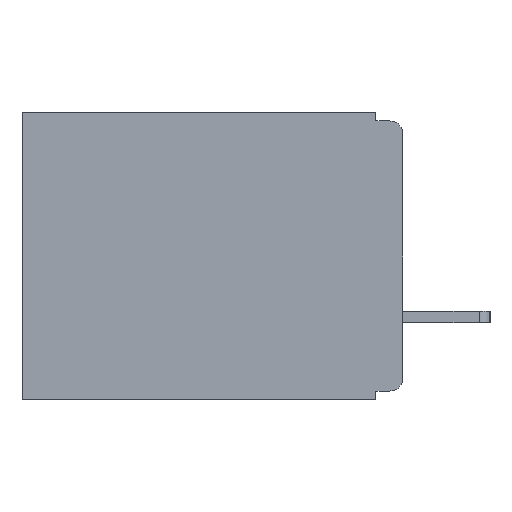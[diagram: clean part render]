
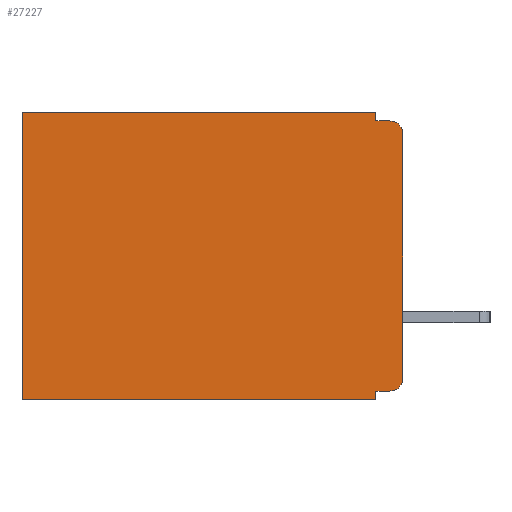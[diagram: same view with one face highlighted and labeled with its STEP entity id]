
A CAD part, left-side view. The second image highlights one B-rep face of the part: STEP entity #27227.
In plain terms, the highlighted planar face has unit normal (-1, 0, 0).
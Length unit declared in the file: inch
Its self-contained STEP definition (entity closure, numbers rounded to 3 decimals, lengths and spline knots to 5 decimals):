
#327 = VERTEX_POINT ( 'NONE', #22125 ) ;
#351 = ORIENTED_EDGE ( 'NONE', *, *, #25943, .F. ) ;
#532 = VERTEX_POINT ( 'NONE', #1681 ) ;
#1321 = VECTOR ( 'NONE', #19471, 39.37008 ) ;
#1681 = CARTESIAN_POINT ( 'NONE',  ( 0.3, 0., -0.025 ) ) ;
#2153 = VECTOR ( 'NONE', #6982, 39.37008 ) ;
#4492 = CARTESIAN_POINT ( 'NONE',  ( 0.3, 0., -0.33 ) ) ;
#4557 = VECTOR ( 'NONE', #11264, 39.37008 ) ;
#4639 = ORIENTED_EDGE ( 'NONE', *, *, #13363, .F. ) ;
#4967 = PLANE ( 'NONE',  #31052 ) ;
#5073 = ORIENTED_EDGE ( 'NONE', *, *, #13217, .F. ) ;
#5121 = DIRECTION ( 'NONE',  ( 0., 0., -1. ) ) ;
#5739 = LINE ( 'NONE', #30008, #31471 ) ;
#6120 = DIRECTION ( 'NONE',  ( -1., 0., 0. ) ) ;
#6982 = DIRECTION ( 'NONE',  ( 0., 0., -1. ) ) ;
#7221 = FACE_OUTER_BOUND ( 'NONE', #11342, .T. ) ;
#7265 = DIRECTION ( 'NONE',  ( 0., 1., 0. ) ) ;
#7323 = LINE ( 'NONE', #23791, #13972 ) ;
#7679 = ORIENTED_EDGE ( 'NONE', *, *, #31259, .F. ) ;
#8275 = CARTESIAN_POINT ( 'NONE',  ( 0.3, 0.031, -0.33 ) ) ;
#8555 = CARTESIAN_POINT ( 'NONE',  ( 0.3, 0.437, 0. ) ) ;
#8827 = CARTESIAN_POINT ( 'NONE',  ( 0.3, 0.437, -0.33 ) ) ;
#8912 = LINE ( 'NONE', #21901, #2153 ) ;
#10006 = DIRECTION ( 'NONE',  ( 0., 0., -1. ) ) ;
#10756 = ORIENTED_EDGE ( 'NONE', *, *, #12569, .T. ) ;
#10912 = ORIENTED_EDGE ( 'NONE', *, *, #28060, .T. ) ;
#11264 = DIRECTION ( 'NONE',  ( 0., 0., -1. ) ) ;
#11342 = EDGE_LOOP ( 'NONE', ( #11739, #31286, #5073, #4639, #10912, #10756, #351, #25464, #7679, #15901 ) ) ;
#11498 = CARTESIAN_POINT ( 'NONE',  ( 0.3, 0., -0.32 ) ) ;
#11739 = ORIENTED_EDGE ( 'NONE', *, *, #13830, .F. ) ;
#12569 = EDGE_CURVE ( 'NONE', #26268, #28171, #24520, .T. ) ;
#13217 = EDGE_CURVE ( 'NONE', #27757, #30675, #7323, .T. ) ;
#13361 = VECTOR ( 'NONE', #16415, 39.37008 ) ;
#13363 = EDGE_CURVE ( 'NONE', #13608, #27757, #8912, .T. ) ;
#13529 = CIRCLE ( 'NONE', #14028, 0.015 ) ;
#13532 = LINE ( 'NONE', #18291, #18556 ) ;
#13608 = VERTEX_POINT ( 'NONE', #18377 ) ;
#13830 = EDGE_CURVE ( 'NONE', #532, #31102, #23732, .T. ) ;
#13834 = AXIS2_PLACEMENT_3D ( 'NONE', #29422, #14460, #31889 ) ;
#13965 = VECTOR ( 'NONE', #7265, 39.37008 ) ;
#13972 = VECTOR ( 'NONE', #18834, 39.37008 ) ;
#14028 = AXIS2_PLACEMENT_3D ( 'NONE', #21052, #6120, #23575 ) ;
#14460 = DIRECTION ( 'NONE',  ( -1., 0., 0. ) ) ;
#15885 = CARTESIAN_POINT ( 'NONE',  ( 0.3, 0., -0.305 ) ) ;
#15901 = ORIENTED_EDGE ( 'NONE', *, *, #21236, .T. ) ;
#16415 = DIRECTION ( 'NONE',  ( 0., 1., 0. ) ) ;
#17143 = CARTESIAN_POINT ( 'NONE',  ( 0.3, 0., -0.33 ) ) ;
#18291 = CARTESIAN_POINT ( 'NONE',  ( 0.3, 0., 0. ) ) ;
#18377 = CARTESIAN_POINT ( 'NONE',  ( 0.3, 0.031, 0. ) ) ;
#18556 = VECTOR ( 'NONE', #23355, 39.37008 ) ;
#18834 = DIRECTION ( 'NONE',  ( 0., -1., 0. ) ) ;
#19154 = CARTESIAN_POINT ( 'NONE',  ( 0.3, 0.015, -0.01 ) ) ;
#19156 = LINE ( 'NONE', #11498, #13361 ) ;
#19471 = DIRECTION ( 'NONE',  ( 0., 0., -1. ) ) ;
#21052 = CARTESIAN_POINT ( 'NONE',  ( 0.3, 0.015, -0.305 ) ) ;
#21203 = CARTESIAN_POINT ( 'NONE',  ( 0.3, 0.437, -0.33 ) ) ;
#21236 = EDGE_CURVE ( 'NONE', #27727, #31102, #13529, .T. ) ;
#21901 = CARTESIAN_POINT ( 'NONE',  ( 0.3, 0.031, 0. ) ) ;
#21933 = EDGE_CURVE ( 'NONE', #532, #30675, #31725, .T. ) ;
#22125 = CARTESIAN_POINT ( 'NONE',  ( 0.3, 0.031, -0.32 ) ) ;
#22445 = CARTESIAN_POINT ( 'NONE',  ( 0.3, 0., -0.33 ) ) ;
#23355 = DIRECTION ( 'NONE',  ( 0., 1., 0. ) ) ;
#23575 = DIRECTION ( 'NONE',  ( 0., 0., -1. ) ) ;
#23732 = LINE ( 'NONE', #4492, #1321 ) ;
#23791 = CARTESIAN_POINT ( 'NONE',  ( 0.3, 0., -0.01 ) ) ;
#24520 = LINE ( 'NONE', #21203, #4557 ) ;
#24962 = DIRECTION ( 'NONE',  ( 1., 0., 0. ) ) ;
#25464 = ORIENTED_EDGE ( 'NONE', *, *, #27863, .F. ) ;
#25943 = EDGE_CURVE ( 'NONE', #31076, #28171, #27212, .T. ) ;
#26268 = VERTEX_POINT ( 'NONE', #8555 ) ;
#27212 = LINE ( 'NONE', #17143, #13965 ) ;
#27227 = ADVANCED_FACE ( 'NONE', ( #7221 ), #4967, .F. ) ;
#27727 = VERTEX_POINT ( 'NONE', #29472 ) ;
#27757 = VERTEX_POINT ( 'NONE', #29582 ) ;
#27863 = EDGE_CURVE ( 'NONE', #327, #31076, #5739, .T. ) ;
#28060 = EDGE_CURVE ( 'NONE', #13608, #26268, #13532, .T. ) ;
#28171 = VERTEX_POINT ( 'NONE', #8827 ) ;
#29422 = CARTESIAN_POINT ( 'NONE',  ( 0.3, 0.015, -0.025 ) ) ;
#29472 = CARTESIAN_POINT ( 'NONE',  ( 0.3, 0.015, -0.32 ) ) ;
#29582 = CARTESIAN_POINT ( 'NONE',  ( 0.3, 0.031, -0.01 ) ) ;
#30008 = CARTESIAN_POINT ( 'NONE',  ( 0.3, 0.031, -0.33 ) ) ;
#30675 = VERTEX_POINT ( 'NONE', #19154 ) ;
#31052 = AXIS2_PLACEMENT_3D ( 'NONE', #22445, #24962, #10006 ) ;
#31076 = VERTEX_POINT ( 'NONE', #8275 ) ;
#31102 = VERTEX_POINT ( 'NONE', #15885 ) ;
#31259 = EDGE_CURVE ( 'NONE', #27727, #327, #19156, .T. ) ;
#31286 = ORIENTED_EDGE ( 'NONE', *, *, #21933, .T. ) ;
#31471 = VECTOR ( 'NONE', #5121, 39.37008 ) ;
#31725 = CIRCLE ( 'NONE', #13834, 0.015 ) ;
#31889 = DIRECTION ( 'NONE',  ( 0., 0., -1. ) ) ;
